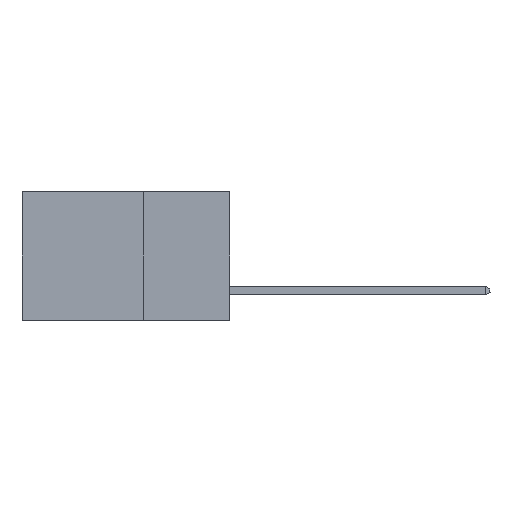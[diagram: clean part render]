
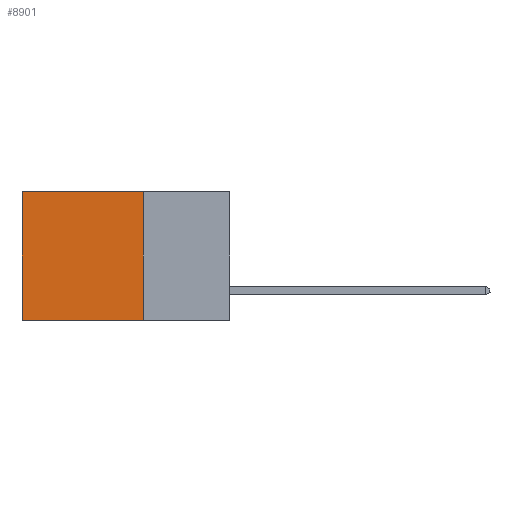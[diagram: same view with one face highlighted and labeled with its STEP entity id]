
A CAD part, left-side view. The second image highlights one B-rep face of the part: STEP entity #8901.
In plain terms, the highlighted planar face has unit normal (-1, 0, 0).
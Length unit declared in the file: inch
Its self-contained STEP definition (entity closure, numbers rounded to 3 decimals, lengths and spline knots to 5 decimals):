
#204 = ORIENTED_EDGE ( 'NONE', *, *, #15177, .F. ) ;
#1622 = LINE ( 'NONE', #8056, #13418 ) ;
#2711 = CARTESIAN_POINT ( 'NONE',  ( 0.298, 0.25, 0. ) ) ;
#2731 = EDGE_CURVE ( 'NONE', #3712, #14324, #9473, .T. ) ;
#2794 = VECTOR ( 'NONE', #17393, 39.37008 ) ;
#2873 = DIRECTION ( 'NONE',  ( 0., 0., -1. ) ) ;
#3487 = EDGE_CURVE ( 'NONE', #13074, #3712, #7712, .T. ) ;
#3712 = VERTEX_POINT ( 'NONE', #11067 ) ;
#4319 = VECTOR ( 'NONE', #12089, 39.37008 ) ;
#4942 = ORIENTED_EDGE ( 'NONE', *, *, #2731, .T. ) ;
#5753 = VECTOR ( 'NONE', #6861, 39.37008 ) ;
#6861 = DIRECTION ( 'NONE',  ( 0., 0., -1. ) ) ;
#7712 = LINE ( 'NONE', #10057, #2794 ) ;
#8056 = CARTESIAN_POINT ( 'NONE',  ( 0.298, 0.25, 0. ) ) ;
#8509 = DIRECTION ( 'NONE',  ( 1., 0., 0. ) ) ;
#8901 = ADVANCED_FACE ( 'NONE', ( #15490 ), #19541, .F. ) ;
#9414 = CARTESIAN_POINT ( 'NONE',  ( 0.298, 0.25, 0. ) ) ;
#9473 = LINE ( 'NONE', #13837, #5753 ) ;
#10057 = CARTESIAN_POINT ( 'NONE',  ( 0.298, 0.25, 0. ) ) ;
#10745 = VERTEX_POINT ( 'NONE', #13983 ) ;
#11067 = CARTESIAN_POINT ( 'NONE',  ( 0.298, 0.6, 0. ) ) ;
#12089 = DIRECTION ( 'NONE',  ( 0., 1., 0. ) ) ;
#12282 = ORIENTED_EDGE ( 'NONE', *, *, #3487, .T. ) ;
#13074 = VERTEX_POINT ( 'NONE', #9414 ) ;
#13195 = DIRECTION ( 'NONE',  ( 0., 0., -1. ) ) ;
#13418 = VECTOR ( 'NONE', #13195, 39.37008 ) ;
#13837 = CARTESIAN_POINT ( 'NONE',  ( 0.298, 0.6, 0. ) ) ;
#13983 = CARTESIAN_POINT ( 'NONE',  ( 0.298, 0.25, -0.37 ) ) ;
#14324 = VERTEX_POINT ( 'NONE', #18278 ) ;
#15177 = EDGE_CURVE ( 'NONE', #10745, #14324, #15305, .T. ) ;
#15305 = LINE ( 'NONE', #22776, #4319 ) ;
#15372 = EDGE_LOOP ( 'NONE', ( #4942, #204, #23247, #12282 ) ) ;
#15490 = FACE_OUTER_BOUND ( 'NONE', #15372, .T. ) ;
#17257 = EDGE_CURVE ( 'NONE', #13074, #10745, #1622, .T. ) ;
#17393 = DIRECTION ( 'NONE',  ( 0., 1., 0. ) ) ;
#18025 = AXIS2_PLACEMENT_3D ( 'NONE', #2711, #8509, #2873 ) ;
#18278 = CARTESIAN_POINT ( 'NONE',  ( 0.298, 0.6, -0.37 ) ) ;
#19541 = PLANE ( 'NONE',  #18025 ) ;
#22776 = CARTESIAN_POINT ( 'NONE',  ( 0.298, 0.25, -0.37 ) ) ;
#23247 = ORIENTED_EDGE ( 'NONE', *, *, #17257, .F. ) ;
